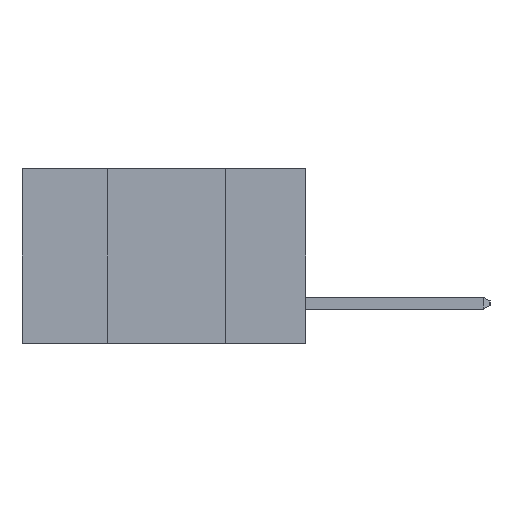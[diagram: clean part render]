
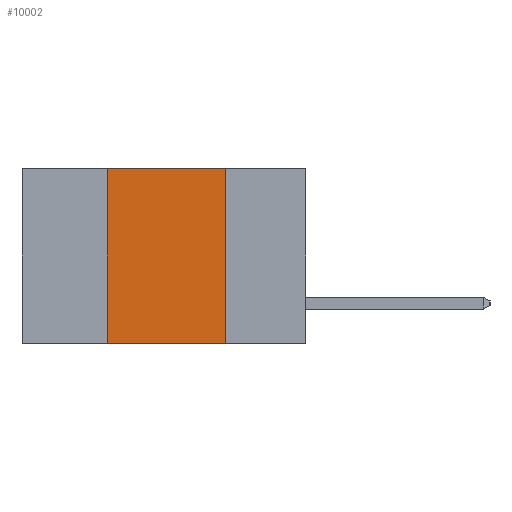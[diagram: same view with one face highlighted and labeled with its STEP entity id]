
A CAD part, left-side view. The second image highlights one B-rep face of the part: STEP entity #10002.
In plain terms, the highlighted planar face has unit normal (-1, 0, 0).
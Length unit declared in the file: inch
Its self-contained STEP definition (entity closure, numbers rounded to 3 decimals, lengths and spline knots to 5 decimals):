
#1007 = VECTOR ( 'NONE', #4784, 39.37008 ) ;
#1401 = CARTESIAN_POINT ( 'NONE',  ( 0., 0.6, -0.37 ) ) ;
#2175 = VERTEX_POINT ( 'NONE', #7989 ) ;
#2678 = VERTEX_POINT ( 'NONE', #13603 ) ;
#2863 = EDGE_LOOP ( 'NONE', ( #11142, #5843, #11492, #3269 ) ) ;
#3160 = VECTOR ( 'NONE', #12574, 39.37008 ) ;
#3269 = ORIENTED_EDGE ( 'NONE', *, *, #9202, .T. ) ;
#3693 = EDGE_CURVE ( 'NONE', #2175, #2678, #8579, .T. ) ;
#3894 = CARTESIAN_POINT ( 'NONE',  ( 0., 0.42, -0.37 ) ) ;
#3963 = PLANE ( 'NONE',  #11388 ) ;
#4350 = VERTEX_POINT ( 'NONE', #8446 ) ;
#4438 = LINE ( 'NONE', #1401, #1007 ) ;
#4784 = DIRECTION ( 'NONE',  ( 0., -1., 0. ) ) ;
#5048 = DIRECTION ( 'NONE',  ( 0., 0., -1. ) ) ;
#5413 = FACE_OUTER_BOUND ( 'NONE', #2863, .T. ) ;
#5843 = ORIENTED_EDGE ( 'NONE', *, *, #6504, .F. ) ;
#6160 = DIRECTION ( 'NONE',  ( 0., -1., 0. ) ) ;
#6188 = CARTESIAN_POINT ( 'NONE',  ( 0., 0.6, 0. ) ) ;
#6340 = LINE ( 'NONE', #6188, #11996 ) ;
#6504 = EDGE_CURVE ( 'NONE', #4350, #2175, #6340, .T. ) ;
#7853 = EDGE_CURVE ( 'NONE', #14009, #4350, #9802, .T. ) ;
#7989 = CARTESIAN_POINT ( 'NONE',  ( 0., 0.17, 0. ) ) ;
#8040 = DIRECTION ( 'NONE',  ( 0., 0., 1. ) ) ;
#8446 = CARTESIAN_POINT ( 'NONE',  ( 0., 0.42, 0. ) ) ;
#8579 = LINE ( 'NONE', #12557, #3160 ) ;
#9202 = EDGE_CURVE ( 'NONE', #14009, #2678, #4438, .T. ) ;
#9802 = LINE ( 'NONE', #10122, #12280 ) ;
#10002 = ADVANCED_FACE ( 'NONE', ( #5413 ), #3963, .F. ) ;
#10122 = CARTESIAN_POINT ( 'NONE',  ( 0., 0.42, -0.37 ) ) ;
#10345 = CARTESIAN_POINT ( 'NONE',  ( 0., 0.6, 0. ) ) ;
#11142 = ORIENTED_EDGE ( 'NONE', *, *, #3693, .F. ) ;
#11388 = AXIS2_PLACEMENT_3D ( 'NONE', #10345, #11414, #5048 ) ;
#11414 = DIRECTION ( 'NONE',  ( 1., 0., 0. ) ) ;
#11492 = ORIENTED_EDGE ( 'NONE', *, *, #7853, .F. ) ;
#11996 = VECTOR ( 'NONE', #6160, 39.37008 ) ;
#12280 = VECTOR ( 'NONE', #8040, 39.37008 ) ;
#12557 = CARTESIAN_POINT ( 'NONE',  ( 0., 0.17, -0.37 ) ) ;
#12574 = DIRECTION ( 'NONE',  ( 0., 0., -1. ) ) ;
#13603 = CARTESIAN_POINT ( 'NONE',  ( 0., 0.17, -0.37 ) ) ;
#14009 = VERTEX_POINT ( 'NONE', #3894 ) ;
